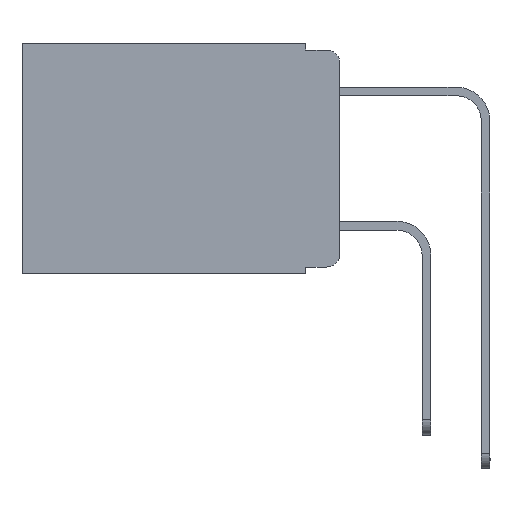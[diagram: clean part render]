
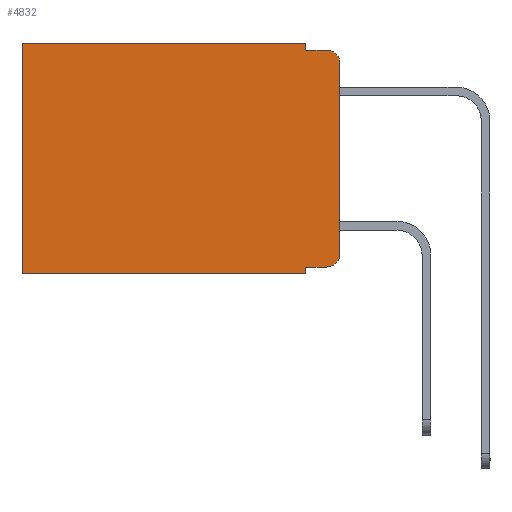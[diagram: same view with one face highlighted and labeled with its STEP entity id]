
A CAD part, left-side view. The second image highlights one B-rep face of the part: STEP entity #4832.
In plain terms, the highlighted planar face has unit normal (-1, 0, 0).
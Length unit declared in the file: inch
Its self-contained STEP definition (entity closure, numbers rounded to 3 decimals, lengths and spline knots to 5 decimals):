
#24 = CARTESIAN_POINT ( 'NONE',  ( 0.298, 0.473, -0.343 ) ) ;
#68 = CIRCLE ( 'NONE', #820, 0.02 ) ;
#131 = VERTEX_POINT ( 'NONE', #11527 ) ;
#400 = DIRECTION ( 'NONE',  ( 0., 0., -1. ) ) ;
#683 = ORIENTED_EDGE ( 'NONE', *, *, #986, .T. ) ;
#820 = AXIS2_PLACEMENT_3D ( 'NONE', #3689, #10938, #11178 ) ;
#986 = EDGE_CURVE ( 'NONE', #9855, #11737, #10334, .T. ) ;
#1174 = EDGE_CURVE ( 'NONE', #1852, #11389, #13647, .T. ) ;
#1205 = CARTESIAN_POINT ( 'NONE',  ( 0.298, 0., -0.343 ) ) ;
#1473 = EDGE_CURVE ( 'NONE', #9855, #9413, #9991, .T. ) ;
#1490 = VECTOR ( 'NONE', #3713, 39.37008 ) ;
#1852 = VERTEX_POINT ( 'NONE', #4616 ) ;
#1875 = VECTOR ( 'NONE', #400, 39.37008 ) ;
#2081 = ORIENTED_EDGE ( 'NONE', *, *, #9530, .T. ) ;
#2117 = ORIENTED_EDGE ( 'NONE', *, *, #6531, .F. ) ;
#2166 = CARTESIAN_POINT ( 'NONE',  ( 0.298, 0.473, 0. ) ) ;
#2222 = LINE ( 'NONE', #8256, #2223 ) ;
#2223 = VECTOR ( 'NONE', #8416, 39.37008 ) ;
#2407 = CARTESIAN_POINT ( 'NONE',  ( 0.298, 0., -0.313 ) ) ;
#2469 = VECTOR ( 'NONE', #9192, 39.37008 ) ;
#2644 = EDGE_CURVE ( 'NONE', #1852, #2903, #15253, .T. ) ;
#2837 = DIRECTION ( 'NONE',  ( 0., 0., -1. ) ) ;
#2845 = CARTESIAN_POINT ( 'NONE',  ( 0.298, 0., 0. ) ) ;
#2903 = VERTEX_POINT ( 'NONE', #12564 ) ;
#2922 = DIRECTION ( 'NONE',  ( 0., 0., -1. ) ) ;
#3380 = EDGE_CURVE ( 'NONE', #2903, #5427, #68, .T. ) ;
#3689 = CARTESIAN_POINT ( 'NONE',  ( 0.298, 0.02, -0.313 ) ) ;
#3713 = DIRECTION ( 'NONE',  ( 0., 0., -1. ) ) ;
#3821 = DIRECTION ( 'NONE',  ( 0., 1., 0. ) ) ;
#3956 = CARTESIAN_POINT ( 'NONE',  ( 0.298, 0.051, -0.01 ) ) ;
#4147 = ORIENTED_EDGE ( 'NONE', *, *, #7993, .F. ) ;
#4389 = ORIENTED_EDGE ( 'NONE', *, *, #7440, .T. ) ;
#4616 = CARTESIAN_POINT ( 'NONE',  ( 0.298, 0.051, -0.333 ) ) ;
#4690 = CARTESIAN_POINT ( 'NONE',  ( 0.298, 0., -0.03 ) ) ;
#4832 = ADVANCED_FACE ( 'NONE', ( #8814 ), #13656, .F. ) ;
#5126 = VERTEX_POINT ( 'NONE', #4690 ) ;
#5137 = ORIENTED_EDGE ( 'NONE', *, *, #2644, .T. ) ;
#5427 = VERTEX_POINT ( 'NONE', #2407 ) ;
#5530 = DIRECTION ( 'NONE',  ( 0., 0., -1. ) ) ;
#6001 = CARTESIAN_POINT ( 'NONE',  ( 0.298, 0.051, -0.343 ) ) ;
#6081 = CARTESIAN_POINT ( 'NONE',  ( 0.298, 0.473, 0. ) ) ;
#6126 = ORIENTED_EDGE ( 'NONE', *, *, #1174, .F. ) ;
#6485 = CARTESIAN_POINT ( 'NONE',  ( 0.298, 0.02, -0.03 ) ) ;
#6531 = EDGE_CURVE ( 'NONE', #5126, #5427, #9113, .T. ) ;
#7147 = CARTESIAN_POINT ( 'NONE',  ( 0.298, 0.051, -0.333 ) ) ;
#7440 = EDGE_CURVE ( 'NONE', #5126, #131, #10247, .T. ) ;
#7465 = VERTEX_POINT ( 'NONE', #24 ) ;
#7549 = CARTESIAN_POINT ( 'NONE',  ( 0.298, 0.051, 0. ) ) ;
#7646 = DIRECTION ( 'NONE',  ( 1., 0., 0. ) ) ;
#7843 = CARTESIAN_POINT ( 'NONE',  ( 0.298, 0.051, 0. ) ) ;
#7993 = EDGE_CURVE ( 'NONE', #9413, #131, #2222, .T. ) ;
#8233 = DIRECTION ( 'NONE',  ( 0., -1., 0. ) ) ;
#8256 = CARTESIAN_POINT ( 'NONE',  ( 0.298, 0.051, -0.01 ) ) ;
#8266 = EDGE_LOOP ( 'NONE', ( #2117, #4389, #4147, #9803, #683, #2081, #10918, #6126, #5137, #13640 ) ) ;
#8416 = DIRECTION ( 'NONE',  ( 0., -1., 0. ) ) ;
#8420 = VECTOR ( 'NONE', #2837, 39.37008 ) ;
#8814 = FACE_OUTER_BOUND ( 'NONE', #8266, .T. ) ;
#9113 = LINE ( 'NONE', #11506, #14758 ) ;
#9180 = EDGE_CURVE ( 'NONE', #11389, #7465, #9692, .T. ) ;
#9192 = DIRECTION ( 'NONE',  ( 0., 1., 0. ) ) ;
#9413 = VERTEX_POINT ( 'NONE', #3956 ) ;
#9530 = EDGE_CURVE ( 'NONE', #11737, #7465, #11984, .T. ) ;
#9692 = LINE ( 'NONE', #1205, #11535 ) ;
#9803 = ORIENTED_EDGE ( 'NONE', *, *, #1473, .F. ) ;
#9855 = VERTEX_POINT ( 'NONE', #7843 ) ;
#9991 = LINE ( 'NONE', #7549, #1875 ) ;
#10247 = CIRCLE ( 'NONE', #12285, 0.02 ) ;
#10334 = LINE ( 'NONE', #13887, #2469 ) ;
#10918 = ORIENTED_EDGE ( 'NONE', *, *, #9180, .F. ) ;
#10938 = DIRECTION ( 'NONE',  ( -1., 0., 0. ) ) ;
#10975 = CARTESIAN_POINT ( 'NONE',  ( 0.298, 0.051, 0. ) ) ;
#10981 = VECTOR ( 'NONE', #8233, 39.37008 ) ;
#11178 = DIRECTION ( 'NONE',  ( 0., 0., -1. ) ) ;
#11389 = VERTEX_POINT ( 'NONE', #6001 ) ;
#11506 = CARTESIAN_POINT ( 'NONE',  ( 0.298, 0., 0. ) ) ;
#11527 = CARTESIAN_POINT ( 'NONE',  ( 0.298, 0.02, -0.01 ) ) ;
#11535 = VECTOR ( 'NONE', #3821, 39.37008 ) ;
#11737 = VERTEX_POINT ( 'NONE', #2166 ) ;
#11984 = LINE ( 'NONE', #6081, #1490 ) ;
#12183 = AXIS2_PLACEMENT_3D ( 'NONE', #2845, #7646, #5530 ) ;
#12285 = AXIS2_PLACEMENT_3D ( 'NONE', #6485, #12639, #2922 ) ;
#12564 = CARTESIAN_POINT ( 'NONE',  ( 0.298, 0.02, -0.333 ) ) ;
#12639 = DIRECTION ( 'NONE',  ( -1., 0., 0. ) ) ;
#13640 = ORIENTED_EDGE ( 'NONE', *, *, #3380, .T. ) ;
#13647 = LINE ( 'NONE', #10975, #8420 ) ;
#13656 = PLANE ( 'NONE',  #12183 ) ;
#13876 = DIRECTION ( 'NONE',  ( 0., 0., -1. ) ) ;
#13887 = CARTESIAN_POINT ( 'NONE',  ( 0.298, 0., 0. ) ) ;
#14758 = VECTOR ( 'NONE', #13876, 39.37008 ) ;
#15253 = LINE ( 'NONE', #7147, #10981 ) ;
